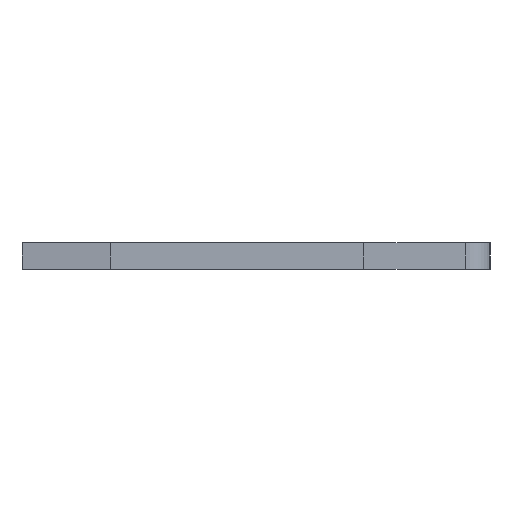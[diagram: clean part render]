
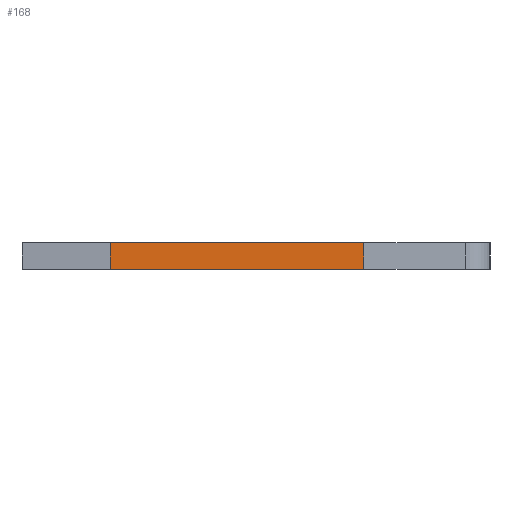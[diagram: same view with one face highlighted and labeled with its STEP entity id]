
A CAD part, left-side view. The second image highlights one B-rep face of the part: STEP entity #168.
In plain terms, the highlighted face is planar.
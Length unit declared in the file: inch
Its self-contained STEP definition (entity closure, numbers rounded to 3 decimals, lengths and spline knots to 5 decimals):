
#4 = FACE_OUTER_BOUND ( 'NONE', #451, .T. ) ;
#9 = LINE ( 'NONE', #290, #408 ) ;
#17 = DIRECTION ( 'NONE',  ( 0., 0., 1. ) ) ;
#35 = DIRECTION ( 'NONE',  ( 0., 1., 0. ) ) ;
#53 = VECTOR ( 'NONE', #71, 39.37008 ) ;
#59 = ORIENTED_EDGE ( 'NONE', *, *, #923, .F. ) ;
#71 = DIRECTION ( 'NONE',  ( -1., 0., 0. ) ) ;
#112 = DIRECTION ( 'NONE',  ( 0., 1., 0. ) ) ;
#125 = VECTOR ( 'NONE', #35, 39.37008 ) ;
#140 = ORIENTED_EDGE ( 'NONE', *, *, #632, .T. ) ;
#168 = ADVANCED_FACE ( 'NONE', ( #4 ), #937, .F. ) ;
#213 = AXIS2_PLACEMENT_3D ( 'NONE', #1045, #17, #759 ) ;
#229 = CARTESIAN_POINT ( 'NONE',  ( 0.013, 0.146, -0.0575 ) ) ;
#275 = VERTEX_POINT ( 'NONE', #327 ) ;
#290 = CARTESIAN_POINT ( 'NONE',  ( 0.013, 0.146, -0.0575 ) ) ;
#292 = DIRECTION ( 'NONE',  ( -1., 0., 0. ) ) ;
#327 = CARTESIAN_POINT ( 'NONE',  ( 0.013, 0.146, -0.0575 ) ) ;
#332 = EDGE_CURVE ( 'NONE', #1079, #275, #758, .T. ) ;
#347 = ORIENTED_EDGE ( 'NONE', *, *, #332, .F. ) ;
#408 = VECTOR ( 'NONE', #292, 39.37008 ) ;
#451 = EDGE_LOOP ( 'NONE', ( #583, #59, #347, #140 ) ) ;
#480 = CARTESIAN_POINT ( 'NONE',  ( 0.013, -0.099, -0.0575 ) ) ;
#515 = LINE ( 'NONE', #530, #53 ) ;
#526 = VERTEX_POINT ( 'NONE', #793 ) ;
#530 = CARTESIAN_POINT ( 'NONE',  ( 0.013, -0.099, -0.0575 ) ) ;
#555 = CARTESIAN_POINT ( 'NONE',  ( -0.013, 0.146, -0.0575 ) ) ;
#583 = ORIENTED_EDGE ( 'NONE', *, *, #1033, .T. ) ;
#589 = LINE ( 'NONE', #555, #1014 ) ;
#632 = EDGE_CURVE ( 'NONE', #1079, #526, #515, .T. ) ;
#758 = LINE ( 'NONE', #229, #125 ) ;
#759 = DIRECTION ( 'NONE',  ( 1., 0., 0. ) ) ;
#793 = CARTESIAN_POINT ( 'NONE',  ( -0.013, -0.099, -0.0575 ) ) ;
#923 = EDGE_CURVE ( 'NONE', #275, #951, #9, .T. ) ;
#929 = CARTESIAN_POINT ( 'NONE',  ( -0.013, 0.146, -0.0575 ) ) ;
#937 = PLANE ( 'NONE',  #213 ) ;
#951 = VERTEX_POINT ( 'NONE', #929 ) ;
#1014 = VECTOR ( 'NONE', #112, 39.37008 ) ;
#1033 = EDGE_CURVE ( 'NONE', #526, #951, #589, .T. ) ;
#1045 = CARTESIAN_POINT ( 'NONE',  ( 0.013, 0.146, -0.0575 ) ) ;
#1079 = VERTEX_POINT ( 'NONE', #480 ) ;
